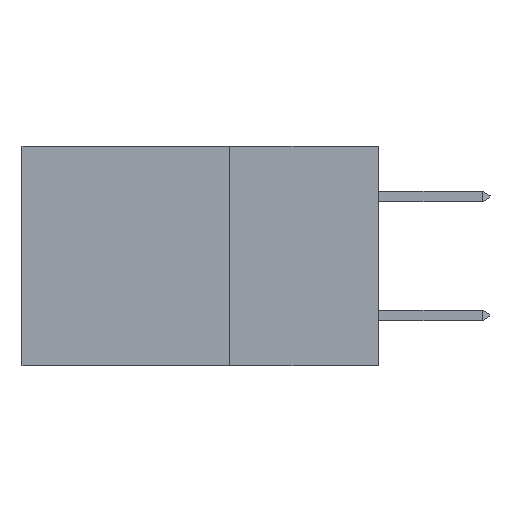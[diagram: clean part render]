
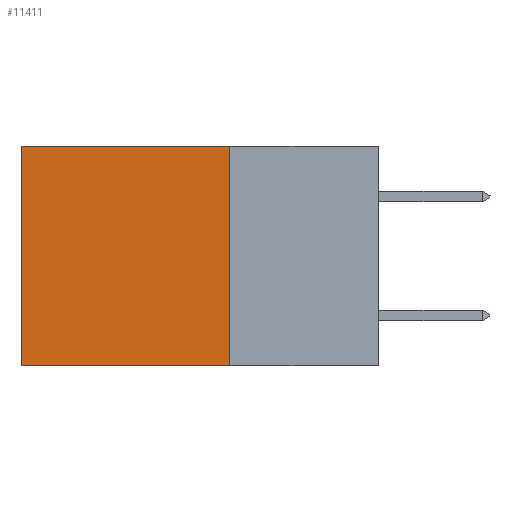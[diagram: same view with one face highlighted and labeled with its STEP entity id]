
A CAD part, left-side view. The second image highlights one B-rep face of the part: STEP entity #11411.
In plain terms, the highlighted planar face has unit normal (-1, 0, 0).
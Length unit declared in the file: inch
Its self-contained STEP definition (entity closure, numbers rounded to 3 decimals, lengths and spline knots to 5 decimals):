
#258 = ORIENTED_EDGE ( 'NONE', *, *, #10146, .T. ) ;
#424 = DIRECTION ( 'NONE',  ( 0., 0., -1. ) ) ;
#532 = VECTOR ( 'NONE', #5616, 39.37008 ) ;
#1041 = EDGE_CURVE ( 'NONE', #14600, #1545, #5379, .T. ) ;
#1374 = CARTESIAN_POINT ( 'NONE',  ( 0.2615, 0.25, -0.37 ) ) ;
#1545 = VERTEX_POINT ( 'NONE', #1374 ) ;
#1689 = PLANE ( 'NONE',  #6775 ) ;
#1777 = CARTESIAN_POINT ( 'NONE',  ( 0.2615, 0.25, -0.37 ) ) ;
#2823 = VERTEX_POINT ( 'NONE', #8133 ) ;
#3401 = DIRECTION ( 'NONE',  ( 0., 1., 0. ) ) ;
#3736 = VECTOR ( 'NONE', #3401, 39.37008 ) ;
#5379 = LINE ( 'NONE', #8935, #7125 ) ;
#5452 = LINE ( 'NONE', #10622, #10507 ) ;
#5616 = DIRECTION ( 'NONE',  ( 0., 0., -1. ) ) ;
#5884 = LINE ( 'NONE', #9767, #3736 ) ;
#6775 = AXIS2_PLACEMENT_3D ( 'NONE', #1777, #11981, #424 ) ;
#7056 = ORIENTED_EDGE ( 'NONE', *, *, #1041, .F. ) ;
#7125 = VECTOR ( 'NONE', #14145, 39.37008 ) ;
#8004 = CARTESIAN_POINT ( 'NONE',  ( 0.2615, 0.25, 0. ) ) ;
#8133 = CARTESIAN_POINT ( 'NONE',  ( 0.2615, 0.6, -0.37 ) ) ;
#8242 = ORIENTED_EDGE ( 'NONE', *, *, #13279, .T. ) ;
#8935 = CARTESIAN_POINT ( 'NONE',  ( 0.2615, 0.25, -0.37 ) ) ;
#9660 = LINE ( 'NONE', #14861, #532 ) ;
#9767 = CARTESIAN_POINT ( 'NONE',  ( 0.2615, 0.25, 0. ) ) ;
#10146 = EDGE_CURVE ( 'NONE', #14600, #13545, #5884, .T. ) ;
#10507 = VECTOR ( 'NONE', #14277, 39.37008 ) ;
#10622 = CARTESIAN_POINT ( 'NONE',  ( 0.2615, 0.25, -0.37 ) ) ;
#11411 = ADVANCED_FACE ( 'NONE', ( #13430 ), #1689, .F. ) ;
#11981 = DIRECTION ( 'NONE',  ( 1., 0., 0. ) ) ;
#13279 = EDGE_CURVE ( 'NONE', #13545, #2823, #9660, .T. ) ;
#13430 = FACE_OUTER_BOUND ( 'NONE', #14740, .T. ) ;
#13545 = VERTEX_POINT ( 'NONE', #14250 ) ;
#14145 = DIRECTION ( 'NONE',  ( 0., 0., -1. ) ) ;
#14250 = CARTESIAN_POINT ( 'NONE',  ( 0.2615, 0.6, 0. ) ) ;
#14277 = DIRECTION ( 'NONE',  ( 0., 1., 0. ) ) ;
#14600 = VERTEX_POINT ( 'NONE', #8004 ) ;
#14740 = EDGE_LOOP ( 'NONE', ( #8242, #14823, #7056, #258 ) ) ;
#14823 = ORIENTED_EDGE ( 'NONE', *, *, #15558, .F. ) ;
#14861 = CARTESIAN_POINT ( 'NONE',  ( 0.2615, 0.6, -0.37 ) ) ;
#15558 = EDGE_CURVE ( 'NONE', #1545, #2823, #5452, .T. ) ;
